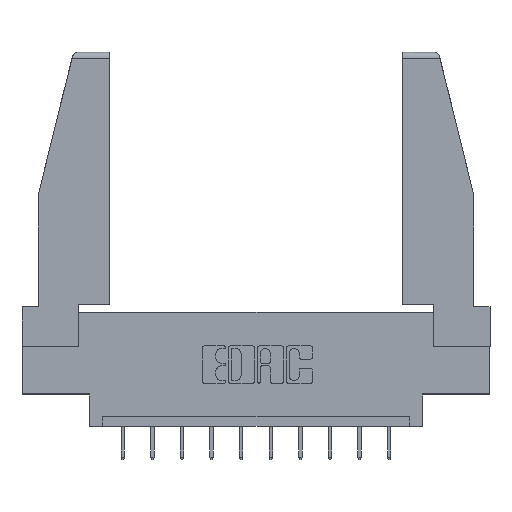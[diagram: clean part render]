
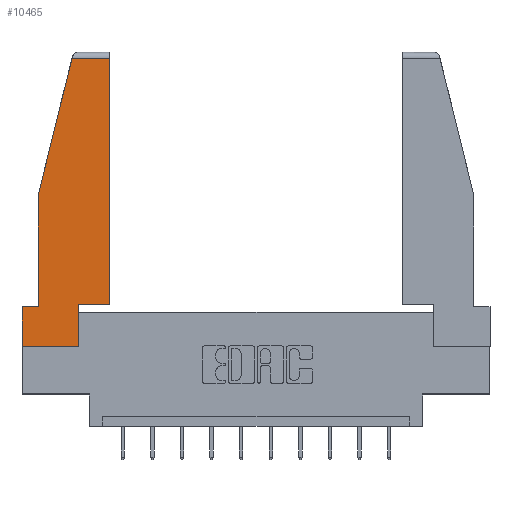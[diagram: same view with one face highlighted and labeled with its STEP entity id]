
A CAD part, top view. The second image highlights one B-rep face of the part: STEP entity #10465.
In plain terms, the highlighted planar face has unit normal (0, 0, 1).
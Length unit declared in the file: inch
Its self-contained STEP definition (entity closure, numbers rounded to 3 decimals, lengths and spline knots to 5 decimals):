
#110 = EDGE_CURVE ( 'NONE', #6704, #7409, #10491, .T. ) ;
#671 = EDGE_CURVE ( 'NONE', #1854, #6704, #12513, .T. ) ;
#1261 = CARTESIAN_POINT ( 'NONE',  ( 0.297, 0.223, 0. ) ) ;
#1289 = CARTESIAN_POINT ( 'NONE',  ( 0., 0.21, 0. ) ) ;
#1854 = VERTEX_POINT ( 'NONE', #14097 ) ;
#2056 = VECTOR ( 'NONE', #4472, 39.37008 ) ;
#2504 = CARTESIAN_POINT ( 'NONE',  ( 0., 0., 0. ) ) ;
#2707 = EDGE_CURVE ( 'NONE', #7409, #8159, #9484, .T. ) ;
#2742 = CARTESIAN_POINT ( 'NONE',  ( 0., 1.52, 0. ) ) ;
#2833 = CARTESIAN_POINT ( 'NONE',  ( 0.461, 0.223, 0. ) ) ;
#3181 = CARTESIAN_POINT ( 'NONE',  ( 0.271, 1.55, 0. ) ) ;
#3656 = CARTESIAN_POINT ( 'NONE',  ( 0.297, 0., 0. ) ) ;
#3859 = VECTOR ( 'NONE', #8948, 39.37008 ) ;
#3877 = ORIENTED_EDGE ( 'NONE', *, *, #671, .T. ) ;
#3880 = LINE ( 'NONE', #11577, #5785 ) ;
#4433 = DIRECTION ( 'NONE',  ( 0., -1., 0. ) ) ;
#4472 = DIRECTION ( 'NONE',  ( -0.239, -0.971, 0. ) ) ;
#4700 = ORIENTED_EDGE ( 'NONE', *, *, #11470, .T. ) ;
#4912 = ORIENTED_EDGE ( 'NONE', *, *, #8025, .T. ) ;
#5032 = LINE ( 'NONE', #3181, #2056 ) ;
#5055 = CARTESIAN_POINT ( 'NONE',  ( 0., 0.21, 0. ) ) ;
#5196 = VERTEX_POINT ( 'NONE', #5055 ) ;
#5409 = FACE_OUTER_BOUND ( 'NONE', #12113, .T. ) ;
#5746 = LINE ( 'NONE', #12004, #8192 ) ;
#5761 = LINE ( 'NONE', #6882, #6651 ) ;
#5785 = VECTOR ( 'NONE', #12539, 39.37008 ) ;
#5795 = ORIENTED_EDGE ( 'NONE', *, *, #110, .T. ) ;
#6002 = PLANE ( 'NONE',  #11774 ) ;
#6061 = VERTEX_POINT ( 'NONE', #8048 ) ;
#6186 = ORIENTED_EDGE ( 'NONE', *, *, #14016, .T. ) ;
#6351 = CARTESIAN_POINT ( 'NONE',  ( 0.461, 1.52, 0. ) ) ;
#6651 = VECTOR ( 'NONE', #11436, 39.37008 ) ;
#6704 = VERTEX_POINT ( 'NONE', #2833 ) ;
#6782 = VECTOR ( 'NONE', #13453, 39.37008 ) ;
#6882 = CARTESIAN_POINT ( 'NONE',  ( 0., 0.21, 0. ) ) ;
#6923 = VECTOR ( 'NONE', #11567, 39.37008 ) ;
#7409 = VERTEX_POINT ( 'NONE', #6351 ) ;
#7467 = ORIENTED_EDGE ( 'NONE', *, *, #2707, .T. ) ;
#7501 = CARTESIAN_POINT ( 'NONE',  ( 0.2636, 1.52, 0. ) ) ;
#8025 = EDGE_CURVE ( 'NONE', #8363, #11990, #10025, .T. ) ;
#8048 = CARTESIAN_POINT ( 'NONE',  ( 0.086, 0.8, 0. ) ) ;
#8159 = VERTEX_POINT ( 'NONE', #7501 ) ;
#8192 = VECTOR ( 'NONE', #4433, 39.37008 ) ;
#8244 = CARTESIAN_POINT ( 'NONE',  ( 0., 0., 0. ) ) ;
#8274 = CARTESIAN_POINT ( 'NONE',  ( 0.086, 0.21, 0. ) ) ;
#8363 = VERTEX_POINT ( 'NONE', #11005 ) ;
#8948 = DIRECTION ( 'NONE',  ( -1., 0., 0. ) ) ;
#9023 = CARTESIAN_POINT ( 'NONE',  ( 0.461, 0.223, 0. ) ) ;
#9070 = DIRECTION ( 'NONE',  ( 0., 1., 0. ) ) ;
#9323 = DIRECTION ( 'NONE',  ( 1., 0., 0. ) ) ;
#9378 = LINE ( 'NONE', #1289, #3859 ) ;
#9484 = LINE ( 'NONE', #2742, #6923 ) ;
#10025 = LINE ( 'NONE', #2504, #6782 ) ;
#10100 = DIRECTION ( 'NONE',  ( 1., 0., 0. ) ) ;
#10189 = EDGE_CURVE ( 'NONE', #12052, #5196, #9378, .T. ) ;
#10351 = EDGE_CURVE ( 'NONE', #5196, #8363, #5761, .T. ) ;
#10411 = DIRECTION ( 'NONE',  ( 0., 0., 1. ) ) ;
#10465 = ADVANCED_FACE ( 'NONE', ( #5409 ), #6002, .T. ) ;
#10489 = EDGE_CURVE ( 'NONE', #6061, #12052, #5746, .T. ) ;
#10491 = LINE ( 'NONE', #9023, #13540 ) ;
#10653 = ORIENTED_EDGE ( 'NONE', *, *, #10351, .T. ) ;
#11005 = CARTESIAN_POINT ( 'NONE',  ( 0., 0., 0. ) ) ;
#11436 = DIRECTION ( 'NONE',  ( 0., -1., 0. ) ) ;
#11439 = ORIENTED_EDGE ( 'NONE', *, *, #10189, .T. ) ;
#11470 = EDGE_CURVE ( 'NONE', #11990, #1854, #3880, .T. ) ;
#11567 = DIRECTION ( 'NONE',  ( -1., 0., 0. ) ) ;
#11577 = CARTESIAN_POINT ( 'NONE',  ( 0.297, 0., 0. ) ) ;
#11774 = AXIS2_PLACEMENT_3D ( 'NONE', #8244, #10411, #9323 ) ;
#11990 = VERTEX_POINT ( 'NONE', #3656 ) ;
#12004 = CARTESIAN_POINT ( 'NONE',  ( 0.086, 0.8, 0. ) ) ;
#12052 = VERTEX_POINT ( 'NONE', #8274 ) ;
#12113 = EDGE_LOOP ( 'NONE', ( #5795, #7467, #6186, #13244, #11439, #10653, #4912, #4700, #3877 ) ) ;
#12513 = LINE ( 'NONE', #1261, #13355 ) ;
#12539 = DIRECTION ( 'NONE',  ( 0., 1., 0. ) ) ;
#13244 = ORIENTED_EDGE ( 'NONE', *, *, #10489, .T. ) ;
#13355 = VECTOR ( 'NONE', #10100, 39.37008 ) ;
#13453 = DIRECTION ( 'NONE',  ( 1., 0., 0. ) ) ;
#13540 = VECTOR ( 'NONE', #9070, 39.37008 ) ;
#14016 = EDGE_CURVE ( 'NONE', #8159, #6061, #5032, .T. ) ;
#14097 = CARTESIAN_POINT ( 'NONE',  ( 0.297, 0.223, 0. ) ) ;
